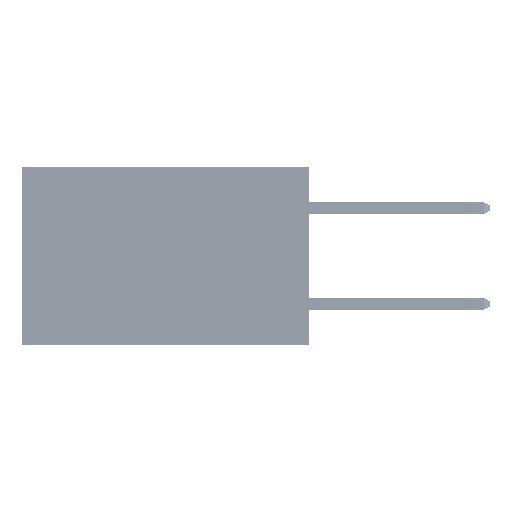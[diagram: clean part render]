
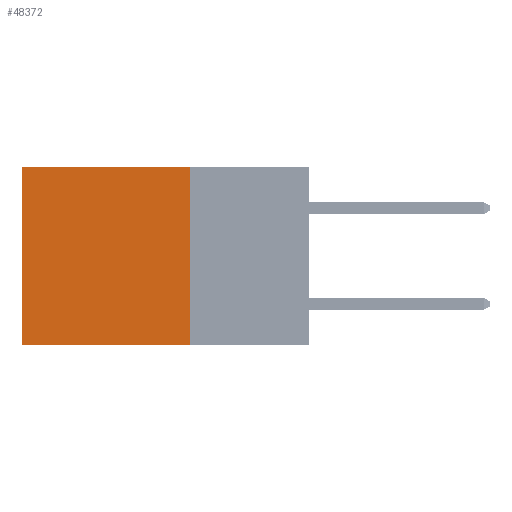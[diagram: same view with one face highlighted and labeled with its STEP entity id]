
A CAD part, left-side view. The second image highlights one B-rep face of the part: STEP entity #48372.
In plain terms, the highlighted planar face has unit normal (-1, 0, 0).
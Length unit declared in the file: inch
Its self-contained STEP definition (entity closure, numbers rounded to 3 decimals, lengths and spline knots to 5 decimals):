
#1462 = EDGE_CURVE ( 'NONE', #39429, #17777, #27721, .T. ) ;
#3082 = ORIENTED_EDGE ( 'NONE', *, *, #30119, .F. ) ;
#3936 = VECTOR ( 'NONE', #32477, 39.37008 ) ;
#5313 = CARTESIAN_POINT ( 'NONE',  ( 0.2875, 0.25, 0. ) ) ;
#6366 = CARTESIAN_POINT ( 'NONE',  ( 0.2875, 0.6, 0. ) ) ;
#7443 = CARTESIAN_POINT ( 'NONE',  ( 0.2875, 0.25, 0. ) ) ;
#10087 = CARTESIAN_POINT ( 'NONE',  ( 0.2875, 0.6, -0.37 ) ) ;
#12087 = CARTESIAN_POINT ( 'NONE',  ( 0.2875, 0.6, 0. ) ) ;
#12393 = VERTEX_POINT ( 'NONE', #7443 ) ;
#17186 = ORIENTED_EDGE ( 'NONE', *, *, #1462, .F. ) ;
#17777 = VERTEX_POINT ( 'NONE', #10087 ) ;
#21414 = LINE ( 'NONE', #5313, #32953 ) ;
#23073 = AXIS2_PLACEMENT_3D ( 'NONE', #31236, #39989, #23725 ) ;
#23725 = DIRECTION ( 'NONE',  ( 0., 0., -1. ) ) ;
#26375 = CARTESIAN_POINT ( 'NONE',  ( 0.2875, 0.25, -0.37 ) ) ;
#26443 = DIRECTION ( 'NONE',  ( 0., 0., -1. ) ) ;
#27721 = LINE ( 'NONE', #49278, #3936 ) ;
#28383 = DIRECTION ( 'NONE',  ( 0., 0., -1. ) ) ;
#29778 = EDGE_CURVE ( 'NONE', #30131, #17777, #35238, .T. ) ;
#29829 = LINE ( 'NONE', #49096, #31726 ) ;
#30119 = EDGE_CURVE ( 'NONE', #12393, #39429, #29829, .T. ) ;
#30131 = VERTEX_POINT ( 'NONE', #12087 ) ;
#31236 = CARTESIAN_POINT ( 'NONE',  ( 0.2875, 0.25, 0. ) ) ;
#31726 = VECTOR ( 'NONE', #28383, 39.37008 ) ;
#32477 = DIRECTION ( 'NONE',  ( 0., 1., 0. ) ) ;
#32558 = ORIENTED_EDGE ( 'NONE', *, *, #29778, .T. ) ;
#32953 = VECTOR ( 'NONE', #38083, 39.37008 ) ;
#35238 = LINE ( 'NONE', #6366, #46719 ) ;
#38083 = DIRECTION ( 'NONE',  ( 0., 1., 0. ) ) ;
#39429 = VERTEX_POINT ( 'NONE', #26375 ) ;
#39989 = DIRECTION ( 'NONE',  ( 1., 0., 0. ) ) ;
#43833 = ORIENTED_EDGE ( 'NONE', *, *, #50641, .T. ) ;
#44262 = PLANE ( 'NONE',  #23073 ) ;
#46194 = EDGE_LOOP ( 'NONE', ( #32558, #17186, #3082, #43833 ) ) ;
#46719 = VECTOR ( 'NONE', #26443, 39.37008 ) ;
#48372 = ADVANCED_FACE ( 'NONE', ( #51094 ), #44262, .F. ) ;
#49096 = CARTESIAN_POINT ( 'NONE',  ( 0.2875, 0.25, 0. ) ) ;
#49278 = CARTESIAN_POINT ( 'NONE',  ( 0.2875, 0.25, -0.37 ) ) ;
#50641 = EDGE_CURVE ( 'NONE', #12393, #30131, #21414, .T. ) ;
#51094 = FACE_OUTER_BOUND ( 'NONE', #46194, .T. ) ;
